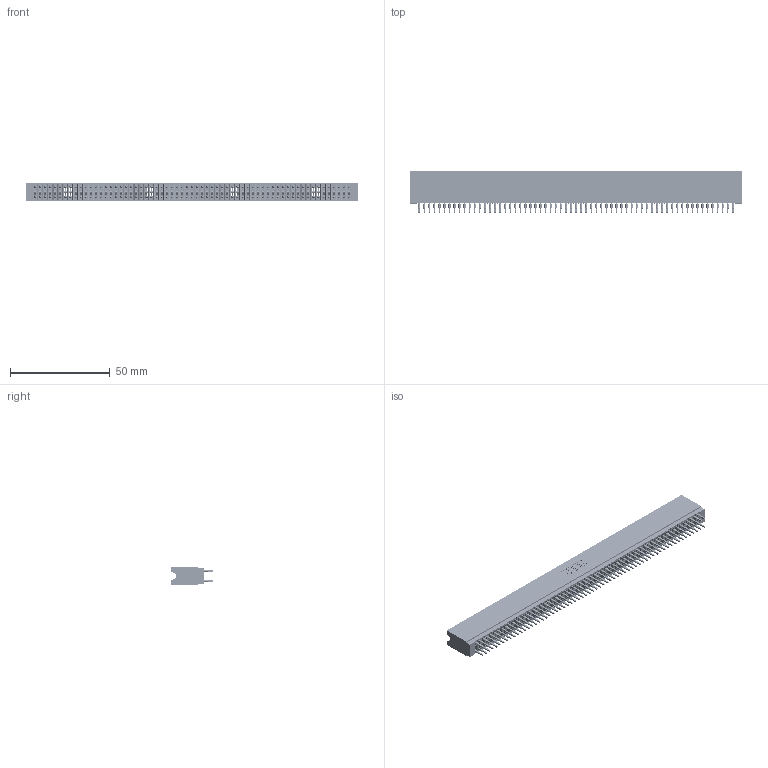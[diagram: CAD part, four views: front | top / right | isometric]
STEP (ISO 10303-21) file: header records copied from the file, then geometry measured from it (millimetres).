
FILE_DESCRIPTION (( 'STEP AP203' ), '1' );
FILE_NAME ('745-126-560-206.STEP', '2026-02-27T02:10:48', ( '' ), ( '' ), 'SwSTEP 2.0', 'SolidWorks 2023', '' );
FILE_SCHEMA (( 'CONFIG_CONTROL_DESIGN' ));
Length unit declared in the file: millimetre
Products named in the file (3): 745-126-560-206; 745 Part_Insulator Option - 06; 745-292-001_560
Assembly tree (127 placements, depth 2):
  745-126-560-206
    745 Part_Insulator Option - 06
    745-292-001_560  x126
Bounding box: 166.62 x 21.22 x 8.89 mm (x, y, z)
Volume: 15322.3 mm3; surface area: 33650.1 mm2
Topology: 127 solids, 127 shells, 12507 faces, 34217 edges, 21718 vertices
Faces by surface type: plane 6482, cylinder 2749, bspline 2520, torus 756
Entity records: 103538 total; most frequent: CARTESIAN_POINT 18456, ORIENTED_EDGE 17934, DIRECTION 15653, EDGE_CURVE 8967, LINE 8399, VECTOR 8399, VERTEX_POINT 5718, AXIS2_PLACEMENT_3D 3627
